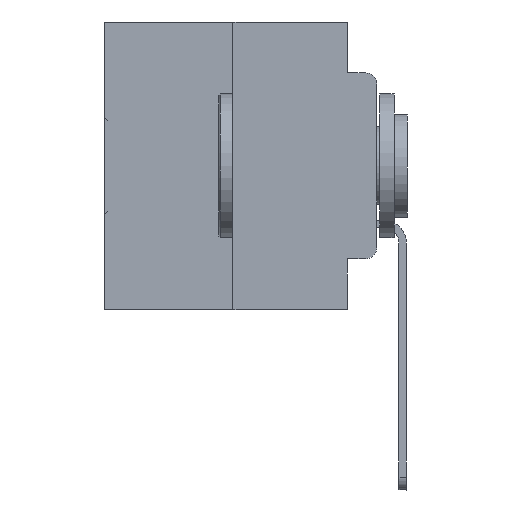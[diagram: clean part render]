
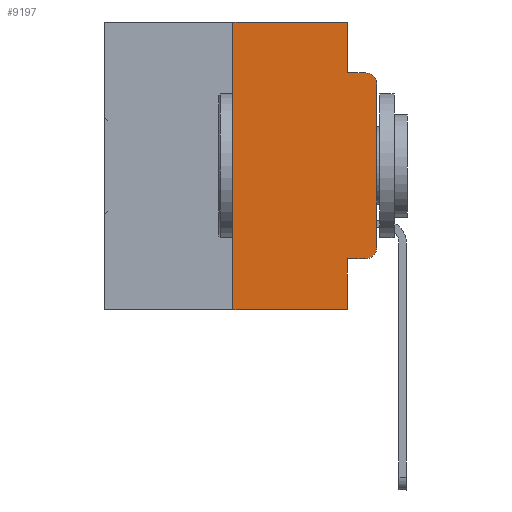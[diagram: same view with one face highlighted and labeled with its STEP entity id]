
A CAD part, left-side view. The second image highlights one B-rep face of the part: STEP entity #9197.
In plain terms, the highlighted planar face has unit normal (-1, 0, 0).
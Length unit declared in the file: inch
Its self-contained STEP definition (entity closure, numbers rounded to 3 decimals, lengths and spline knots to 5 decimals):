
#130 = CARTESIAN_POINT ( 'NONE',  ( 0., 0.051, -0.4115 ) ) ;
#131 = DIRECTION ( 'NONE',  ( 1., 0., 0. ) ) ;
#634 = VECTOR ( 'NONE', #23104, 39.37008 ) ;
#978 = CARTESIAN_POINT ( 'NONE',  ( 0., 0., -0.1085 ) ) ;
#1295 = VECTOR ( 'NONE', #22513, 39.37008 ) ;
#1582 = CARTESIAN_POINT ( 'NONE',  ( 0., 0.051, -0.4115 ) ) ;
#1865 = VERTEX_POINT ( 'NONE', #130 ) ;
#2182 = VECTOR ( 'NONE', #7592, 39.37008 ) ;
#2489 = DIRECTION ( 'NONE',  ( 0., 0., -1. ) ) ;
#2588 = VECTOR ( 'NONE', #3444, 39.37008 ) ;
#2892 = LINE ( 'NONE', #12988, #634 ) ;
#2941 = DIRECTION ( 'NONE',  ( 0., 0., -1. ) ) ;
#3444 = DIRECTION ( 'NONE',  ( 0., 0., 1. ) ) ;
#3595 = ORIENTED_EDGE ( 'NONE', *, *, #27911, .F. ) ;
#4465 = LINE ( 'NONE', #27181, #1295 ) ;
#4502 = CARTESIAN_POINT ( 'NONE',  ( 0., 0.051, 0. ) ) ;
#4586 = EDGE_CURVE ( 'NONE', #23294, #5807, #24659, .T. ) ;
#4832 = LINE ( 'NONE', #30353, #31482 ) ;
#5190 = EDGE_CURVE ( 'NONE', #23900, #27259, #2892, .T. ) ;
#5346 = CIRCLE ( 'NONE', #6416, 0.02 ) ;
#5807 = VERTEX_POINT ( 'NONE', #4502 ) ;
#6416 = AXIS2_PLACEMENT_3D ( 'NONE', #13619, #23914, #18427 ) ;
#6751 = CARTESIAN_POINT ( 'NONE',  ( 0., 0.25, 0. ) ) ;
#6870 = CARTESIAN_POINT ( 'NONE',  ( 0., 0.02, -0.4115 ) ) ;
#7480 = LINE ( 'NONE', #17564, #29074 ) ;
#7592 = DIRECTION ( 'NONE',  ( 0., -1., 0. ) ) ;
#7713 = VECTOR ( 'NONE', #19156, 39.37008 ) ;
#8248 = EDGE_CURVE ( 'NONE', #1865, #28147, #16330, .T. ) ;
#8447 = AXIS2_PLACEMENT_3D ( 'NONE', #11695, #29460, #17161 ) ;
#9197 = ADVANCED_FACE ( 'NONE', ( #15687 ), #15210, .F. ) ;
#10716 = EDGE_LOOP ( 'NONE', ( #14606, #18826, #3595, #16270, #28810, #19941, #32766, #27234, #30912, #29932 ) ) ;
#11497 = EDGE_CURVE ( 'NONE', #23900, #23294, #29473, .T. ) ;
#11695 = CARTESIAN_POINT ( 'NONE',  ( 0., 0.02, -0.3915 ) ) ;
#12988 = CARTESIAN_POINT ( 'NONE',  ( 0., 0.473, -0.5 ) ) ;
#12991 = VERTEX_POINT ( 'NONE', #13330 ) ;
#13126 = CARTESIAN_POINT ( 'NONE',  ( 0., 0.25, -0.5 ) ) ;
#13330 = CARTESIAN_POINT ( 'NONE',  ( 0., 0.02, -0.0885 ) ) ;
#13619 = CARTESIAN_POINT ( 'NONE',  ( 0., 0.02, -0.1085 ) ) ;
#13806 = VERTEX_POINT ( 'NONE', #22067 ) ;
#14606 = ORIENTED_EDGE ( 'NONE', *, *, #31424, .T. ) ;
#14768 = CARTESIAN_POINT ( 'NONE',  ( 0., 0., 0. ) ) ;
#15153 = CARTESIAN_POINT ( 'NONE',  ( 0., 0., -0.3915 ) ) ;
#15210 = PLANE ( 'NONE',  #27456 ) ;
#15424 = LINE ( 'NONE', #14768, #25224 ) ;
#15687 = FACE_OUTER_BOUND ( 'NONE', #10716, .T. ) ;
#16270 = ORIENTED_EDGE ( 'NONE', *, *, #27472, .F. ) ;
#16330 = LINE ( 'NONE', #1582, #7713 ) ;
#17161 = DIRECTION ( 'NONE',  ( 0., 0., -1. ) ) ;
#17564 = CARTESIAN_POINT ( 'NONE',  ( 0., 0.051, 0. ) ) ;
#18427 = DIRECTION ( 'NONE',  ( 0., 0., -1. ) ) ;
#18826 = ORIENTED_EDGE ( 'NONE', *, *, #22772, .T. ) ;
#19156 = DIRECTION ( 'NONE',  ( 0., -1., 0. ) ) ;
#19834 = CARTESIAN_POINT ( 'NONE',  ( 0., 0.25, 0. ) ) ;
#19941 = ORIENTED_EDGE ( 'NONE', *, *, #11497, .F. ) ;
#20219 = EDGE_CURVE ( 'NONE', #28147, #31986, #28553, .T. ) ;
#21141 = EDGE_CURVE ( 'NONE', #1865, #27259, #7480, .T. ) ;
#22067 = CARTESIAN_POINT ( 'NONE',  ( 0., 0.051, -0.0885 ) ) ;
#22513 = DIRECTION ( 'NONE',  ( 0., -1., 0. ) ) ;
#22772 = EDGE_CURVE ( 'NONE', #28915, #12991, #5346, .T. ) ;
#23104 = DIRECTION ( 'NONE',  ( 0., -1., 0. ) ) ;
#23294 = VERTEX_POINT ( 'NONE', #19834 ) ;
#23900 = VERTEX_POINT ( 'NONE', #13126 ) ;
#23914 = DIRECTION ( 'NONE',  ( -1., 0., 0. ) ) ;
#24659 = LINE ( 'NONE', #24811, #2182 ) ;
#24811 = CARTESIAN_POINT ( 'NONE',  ( 0., 0.473, 0. ) ) ;
#25224 = VECTOR ( 'NONE', #30206, 39.37008 ) ;
#27181 = CARTESIAN_POINT ( 'NONE',  ( 0., 0.051, -0.0885 ) ) ;
#27234 = ORIENTED_EDGE ( 'NONE', *, *, #21141, .F. ) ;
#27259 = VERTEX_POINT ( 'NONE', #30701 ) ;
#27456 = AXIS2_PLACEMENT_3D ( 'NONE', #27825, #131, #2941 ) ;
#27472 = EDGE_CURVE ( 'NONE', #5807, #13806, #4832, .T. ) ;
#27825 = CARTESIAN_POINT ( 'NONE',  ( 0., 0.473, 0. ) ) ;
#27911 = EDGE_CURVE ( 'NONE', #13806, #12991, #4465, .T. ) ;
#28147 = VERTEX_POINT ( 'NONE', #6870 ) ;
#28553 = CIRCLE ( 'NONE', #8447, 0.02 ) ;
#28810 = ORIENTED_EDGE ( 'NONE', *, *, #4586, .F. ) ;
#28915 = VERTEX_POINT ( 'NONE', #978 ) ;
#29074 = VECTOR ( 'NONE', #32352, 39.37008 ) ;
#29460 = DIRECTION ( 'NONE',  ( -1., 0., 0. ) ) ;
#29473 = LINE ( 'NONE', #6751, #2588 ) ;
#29932 = ORIENTED_EDGE ( 'NONE', *, *, #20219, .T. ) ;
#30206 = DIRECTION ( 'NONE',  ( 0., 0., 1. ) ) ;
#30353 = CARTESIAN_POINT ( 'NONE',  ( 0., 0.051, 0. ) ) ;
#30701 = CARTESIAN_POINT ( 'NONE',  ( 0., 0.051, -0.5 ) ) ;
#30912 = ORIENTED_EDGE ( 'NONE', *, *, #8248, .T. ) ;
#31424 = EDGE_CURVE ( 'NONE', #31986, #28915, #15424, .T. ) ;
#31482 = VECTOR ( 'NONE', #2489, 39.37008 ) ;
#31986 = VERTEX_POINT ( 'NONE', #15153 ) ;
#32352 = DIRECTION ( 'NONE',  ( 0., 0., -1. ) ) ;
#32766 = ORIENTED_EDGE ( 'NONE', *, *, #5190, .T. ) ;
